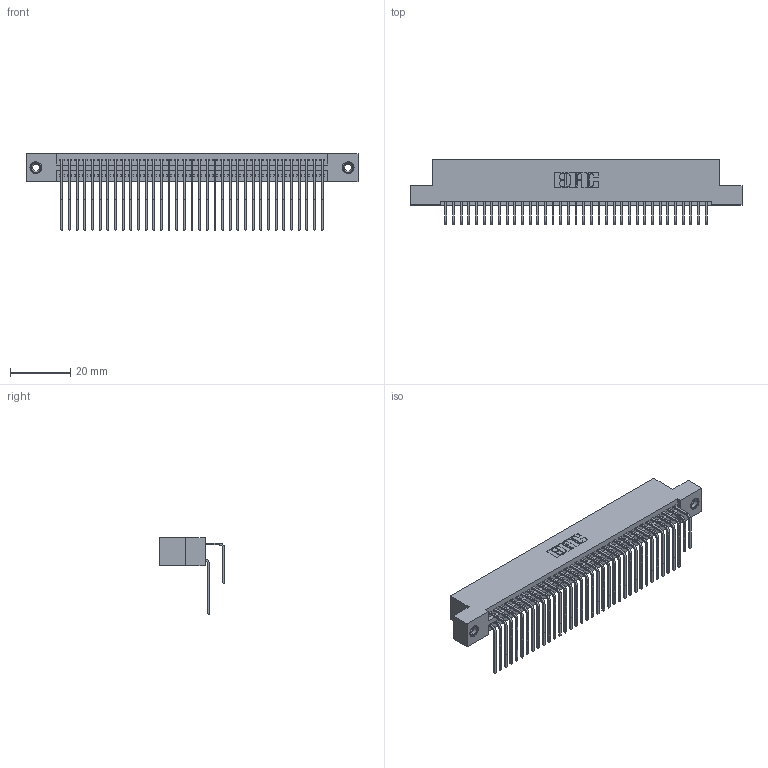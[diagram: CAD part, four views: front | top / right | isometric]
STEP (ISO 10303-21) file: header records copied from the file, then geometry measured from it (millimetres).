
FILE_DESCRIPTION (( 'STEP AP203' ), '1' );
FILE_NAME ('345-070-558-208.STEP', '2018-10-01T10:01:17', ( '' ), ( '' ), 'SwSTEP 2.0', 'SolidWorks 2016', '' );
FILE_SCHEMA (( 'CONFIG_CONTROL_DESIGN' ));
Length unit declared in the file: inch
Products named in the file (5): 345-250-001_345-250-003-102; 345-292-001_558 559 Tail - 1; 345 Part_Flush Mounting Lugs - 0.156 Dia-TI; 345-070-558-208; 345-292-001_558 Tail - 2
Assembly tree (73 placements, depth 2):
  345-070-558-208
    345 Part_Flush Mounting Lugs - 0.156 Dia-TI
    345-292-001_558 559 Tail - 1  x35
    345-292-001_558 Tail - 2  x35
    345-250-001_345-250-003-102  x2
Bounding box: 110.11 x 21.83 x 25.53 mm (x, y, z)
Volume: 11028.4 mm3; surface area: 18078.6 mm2
Topology: 73 solids, 73 shells, 3826 faces, 11327 edges, 7450 vertices
Faces by surface type: plane 2562, cylinder 1248, cone 12, torus 4
Entity records: 31242 total; most frequent: CARTESIAN_POINT 5270, ORIENTED_EDGE 5146, DIRECTION 4655, EDGE_CURVE 2573, VECTOR 2241, LINE 2241, VERTEX_POINT 1708, AXIS2_PLACEMENT_3D 1207
